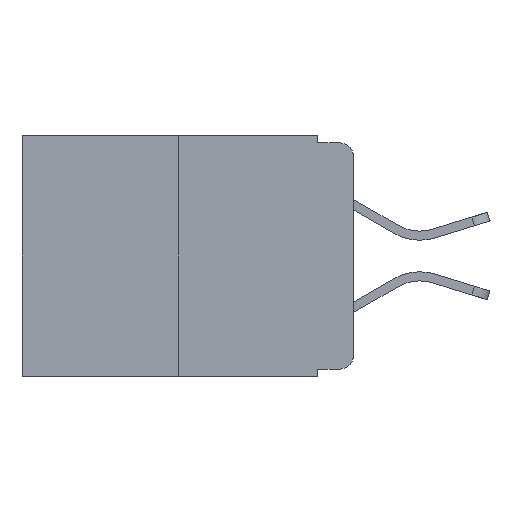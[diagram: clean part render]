
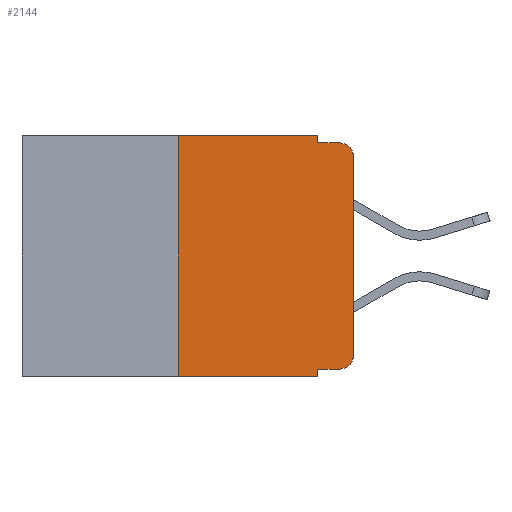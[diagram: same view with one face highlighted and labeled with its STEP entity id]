
A CAD part, left-side view. The second image highlights one B-rep face of the part: STEP entity #2144.
In plain terms, the highlighted planar face has unit normal (-1, 0, 0).
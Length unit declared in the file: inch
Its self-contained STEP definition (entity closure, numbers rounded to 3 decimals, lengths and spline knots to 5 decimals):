
#48 = DIRECTION ( 'NONE',  ( 0., 0., -1. ) ) ;
#59 = EDGE_CURVE ( 'NONE', #4526, #10546, #6197, .T. ) ;
#154 = VERTEX_POINT ( 'NONE', #6068 ) ;
#502 = CARTESIAN_POINT ( 'NONE',  ( 0., 0.25, -0.343 ) ) ;
#602 = VECTOR ( 'NONE', #7045, 39.37008 ) ;
#673 = ORIENTED_EDGE ( 'NONE', *, *, #10045, .T. ) ;
#711 = LINE ( 'NONE', #10904, #7380 ) ;
#731 = AXIS2_PLACEMENT_3D ( 'NONE', #2279, #10540, #48 ) ;
#735 = CARTESIAN_POINT ( 'NONE',  ( 0., 0.02, -0.03 ) ) ;
#1189 = VERTEX_POINT ( 'NONE', #4184 ) ;
#1193 = DIRECTION ( 'NONE',  ( 0., -1., 0. ) ) ;
#1377 = CARTESIAN_POINT ( 'NONE',  ( 0., 0.02, -0.313 ) ) ;
#1620 = VECTOR ( 'NONE', #6013, 39.37008 ) ;
#1645 = CARTESIAN_POINT ( 'NONE',  ( 0., 0.051, -0.01 ) ) ;
#1669 = DIRECTION ( 'NONE',  ( 0., 0., -1. ) ) ;
#1729 = CARTESIAN_POINT ( 'NONE',  ( 0., 0.25, 0. ) ) ;
#1826 = CARTESIAN_POINT ( 'NONE',  ( 0., 0.051, 0. ) ) ;
#1953 = PLANE ( 'NONE',  #731 ) ;
#2061 = VERTEX_POINT ( 'NONE', #1729 ) ;
#2144 = ADVANCED_FACE ( 'NONE', ( #9390 ), #1953, .F. ) ;
#2279 = CARTESIAN_POINT ( 'NONE',  ( 0., 0.473, 0. ) ) ;
#2318 = DIRECTION ( 'NONE',  ( 0., 0., -1. ) ) ;
#2342 = ORIENTED_EDGE ( 'NONE', *, *, #4148, .T. ) ;
#2553 = ORIENTED_EDGE ( 'NONE', *, *, #7421, .T. ) ;
#2726 = ORIENTED_EDGE ( 'NONE', *, *, #8465, .F. ) ;
#2765 = CARTESIAN_POINT ( 'NONE',  ( 0., 0., 0. ) ) ;
#2959 = CARTESIAN_POINT ( 'NONE',  ( 0., 0., -0.313 ) ) ;
#3028 = CARTESIAN_POINT ( 'NONE',  ( 0., 0.473, 0. ) ) ;
#3048 = LINE ( 'NONE', #5266, #602 ) ;
#3052 = CARTESIAN_POINT ( 'NONE',  ( 0., 0.02, -0.01 ) ) ;
#3066 = AXIS2_PLACEMENT_3D ( 'NONE', #1377, #7693, #2318 ) ;
#3072 = EDGE_LOOP ( 'NONE', ( #3228, #3481, #4319, #4680, #4961, #6195, #2553, #2726, #673, #2342 ) ) ;
#3122 = DIRECTION ( 'NONE',  ( 0., -1., 0. ) ) ;
#3158 = CARTESIAN_POINT ( 'NONE',  ( 0., 0.051, -0.343 ) ) ;
#3228 = ORIENTED_EDGE ( 'NONE', *, *, #59, .T. ) ;
#3481 = ORIENTED_EDGE ( 'NONE', *, *, #4378, .T. ) ;
#3588 = DIRECTION ( 'NONE',  ( 0., -1., 0. ) ) ;
#3589 = VECTOR ( 'NONE', #3122, 39.37008 ) ;
#4148 = EDGE_CURVE ( 'NONE', #1189, #4526, #9961, .T. ) ;
#4184 = CARTESIAN_POINT ( 'NONE',  ( 0., 0.02, -0.333 ) ) ;
#4319 = ORIENTED_EDGE ( 'NONE', *, *, #5594, .F. ) ;
#4378 = EDGE_CURVE ( 'NONE', #10546, #7016, #6398, .T. ) ;
#4526 = VERTEX_POINT ( 'NONE', #2959 ) ;
#4648 = DIRECTION ( 'NONE',  ( 0., -1., 0. ) ) ;
#4680 = ORIENTED_EDGE ( 'NONE', *, *, #5000, .F. ) ;
#4882 = CARTESIAN_POINT ( 'NONE',  ( 0., 0., -0.03 ) ) ;
#4961 = ORIENTED_EDGE ( 'NONE', *, *, #5248, .F. ) ;
#5000 = EDGE_CURVE ( 'NONE', #6410, #5523, #6670, .T. ) ;
#5248 = EDGE_CURVE ( 'NONE', #2061, #6410, #6801, .T. ) ;
#5266 = CARTESIAN_POINT ( 'NONE',  ( 0., 0.051, 0. ) ) ;
#5523 = VERTEX_POINT ( 'NONE', #1645 ) ;
#5594 = EDGE_CURVE ( 'NONE', #5523, #7016, #9960, .T. ) ;
#5719 = LINE ( 'NONE', #8409, #3589 ) ;
#6013 = DIRECTION ( 'NONE',  ( 0., 0., 1. ) ) ;
#6068 = CARTESIAN_POINT ( 'NONE',  ( 0., 0.051, -0.333 ) ) ;
#6069 = VERTEX_POINT ( 'NONE', #502 ) ;
#6127 = AXIS2_PLACEMENT_3D ( 'NONE', #735, #7101, #1669 ) ;
#6195 = ORIENTED_EDGE ( 'NONE', *, *, #9530, .F. ) ;
#6197 = LINE ( 'NONE', #2765, #1620 ) ;
#6398 = CIRCLE ( 'NONE', #6127, 0.02 ) ;
#6410 = VERTEX_POINT ( 'NONE', #7277 ) ;
#6655 = VERTEX_POINT ( 'NONE', #3158 ) ;
#6670 = LINE ( 'NONE', #1826, #6940 ) ;
#6801 = LINE ( 'NONE', #3028, #7066 ) ;
#6912 = DIRECTION ( 'NONE',  ( 0., 0., 1. ) ) ;
#6940 = VECTOR ( 'NONE', #10437, 39.37008 ) ;
#7016 = VERTEX_POINT ( 'NONE', #3052 ) ;
#7045 = DIRECTION ( 'NONE',  ( 0., 0., -1. ) ) ;
#7066 = VECTOR ( 'NONE', #1193, 39.37008 ) ;
#7101 = DIRECTION ( 'NONE',  ( -1., 0., 0. ) ) ;
#7277 = CARTESIAN_POINT ( 'NONE',  ( 0., 0.051, 0. ) ) ;
#7380 = VECTOR ( 'NONE', #6912, 39.37008 ) ;
#7421 = EDGE_CURVE ( 'NONE', #6069, #6655, #10057, .T. ) ;
#7693 = DIRECTION ( 'NONE',  ( -1., 0., 0. ) ) ;
#7935 = VECTOR ( 'NONE', #4648, 39.37008 ) ;
#8409 = CARTESIAN_POINT ( 'NONE',  ( 0., 0.051, -0.333 ) ) ;
#8465 = EDGE_CURVE ( 'NONE', #154, #6655, #3048, .T. ) ;
#9390 = FACE_OUTER_BOUND ( 'NONE', #3072, .T. ) ;
#9530 = EDGE_CURVE ( 'NONE', #6069, #2061, #711, .T. ) ;
#9724 = CARTESIAN_POINT ( 'NONE',  ( 0., 0.473, -0.343 ) ) ;
#9856 = VECTOR ( 'NONE', #3588, 39.37008 ) ;
#9960 = LINE ( 'NONE', #11141, #9856 ) ;
#9961 = CIRCLE ( 'NONE', #3066, 0.02 ) ;
#10045 = EDGE_CURVE ( 'NONE', #154, #1189, #5719, .T. ) ;
#10057 = LINE ( 'NONE', #9724, #7935 ) ;
#10437 = DIRECTION ( 'NONE',  ( 0., 0., -1. ) ) ;
#10540 = DIRECTION ( 'NONE',  ( 1., 0., 0. ) ) ;
#10546 = VERTEX_POINT ( 'NONE', #4882 ) ;
#10904 = CARTESIAN_POINT ( 'NONE',  ( 0., 0.25, 0. ) ) ;
#11141 = CARTESIAN_POINT ( 'NONE',  ( 0., 0.051, -0.01 ) ) ;
